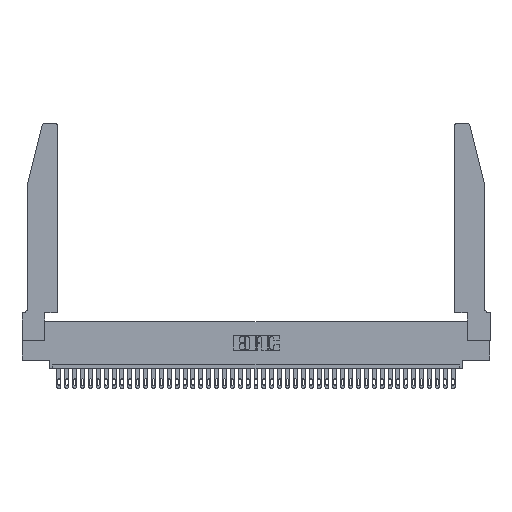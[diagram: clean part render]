
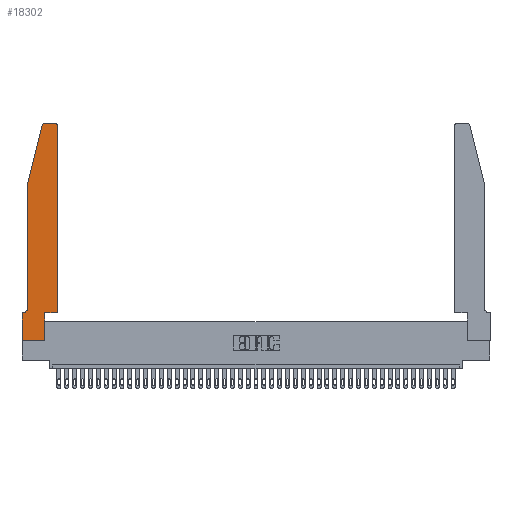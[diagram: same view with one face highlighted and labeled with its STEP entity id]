
A CAD part, top view. The second image highlights one B-rep face of the part: STEP entity #18302.
In plain terms, the highlighted planar face has unit normal (0, 0, 1).
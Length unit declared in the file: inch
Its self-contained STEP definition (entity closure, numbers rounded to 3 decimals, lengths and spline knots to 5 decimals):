
#527 = CARTESIAN_POINT ( 'NONE',  ( 0.0755, 2., 0.37 ) ) ;
#579 = DIRECTION ( 'NONE',  ( 1., 0., 0. ) ) ;
#668 = DIRECTION ( 'NONE',  ( -0.239, -0.971, 0. ) ) ;
#1017 = LINE ( 'NONE', #32076, #15274 ) ;
#1327 = VERTEX_POINT ( 'NONE', #15235 ) ;
#2550 = CIRCLE ( 'NONE', #15860, 0.07 ) ;
#3714 = VECTOR ( 'NONE', #8068, 39.37008 ) ;
#3719 = EDGE_CURVE ( 'NONE', #20723, #32697, #11274, .T. ) ;
#4238 = VERTEX_POINT ( 'NONE', #23955 ) ;
#4839 = EDGE_CURVE ( 'NONE', #19956, #35145, #35488, .T. ) ;
#6407 = VERTEX_POINT ( 'NONE', #12222 ) ;
#6591 = DIRECTION ( 'NONE',  ( 1., 0., 0. ) ) ;
#6674 = ORIENTED_EDGE ( 'NONE', *, *, #29566, .T. ) ;
#7957 = FACE_OUTER_BOUND ( 'NONE', #36875, .T. ) ;
#8068 = DIRECTION ( 'NONE',  ( 0., -1., 0. ) ) ;
#8104 = ORIENTED_EDGE ( 'NONE', *, *, #24002, .T. ) ;
#8950 = EDGE_CURVE ( 'NONE', #16561, #6407, #25975, .T. ) ;
#9251 = CARTESIAN_POINT ( 'NONE',  ( 0., 0.35, 0.37 ) ) ;
#9753 = ORIENTED_EDGE ( 'NONE', *, *, #22561, .T. ) ;
#11274 = LINE ( 'NONE', #40471, #36041 ) ;
#12089 = DIRECTION ( 'NONE',  ( 1., 0., 0. ) ) ;
#12222 = CARTESIAN_POINT ( 'NONE',  ( 0.0755, 2., 0.37 ) ) ;
#14002 = CARTESIAN_POINT ( 'NONE',  ( 0., 0.35, 0.37 ) ) ;
#14170 = LINE ( 'NONE', #36055, #40534 ) ;
#14314 = CIRCLE ( 'NONE', #27351, 0.03 ) ;
#14444 = ORIENTED_EDGE ( 'NONE', *, *, #4839, .T. ) ;
#14509 = DIRECTION ( 'NONE',  ( 0., 1., 0. ) ) ;
#14653 = CARTESIAN_POINT ( 'NONE',  ( 0.284, 2.75, 0.37 ) ) ;
#14959 = ORIENTED_EDGE ( 'NONE', *, *, #37560, .T. ) ;
#15235 = CARTESIAN_POINT ( 'NONE',  ( 0.0055, 0.35, 0.37 ) ) ;
#15274 = VECTOR ( 'NONE', #31943, 39.37008 ) ;
#15860 = AXIS2_PLACEMENT_3D ( 'NONE', #17059, #26700, #26286 ) ;
#16427 = PLANE ( 'NONE',  #25209 ) ;
#16561 = VERTEX_POINT ( 'NONE', #34721 ) ;
#16781 = AXIS2_PLACEMENT_3D ( 'NONE', #28694, #24999, #24856 ) ;
#17059 = CARTESIAN_POINT ( 'NONE',  ( 0.0055, 0.42, 0.37 ) ) ;
#18076 = CARTESIAN_POINT ( 'NONE',  ( 0.0755, 0.42, 0.37 ) ) ;
#18302 = ADVANCED_FACE ( 'NONE', ( #7957 ), #16427, .T. ) ;
#18661 = DIRECTION ( 'NONE',  ( -1., 0., 0. ) ) ;
#19955 = VERTEX_POINT ( 'NONE', #18076 ) ;
#19956 = VERTEX_POINT ( 'NONE', #31541 ) ;
#19989 = CARTESIAN_POINT ( 'NONE',  ( 0.4205, 2.72, 0.37 ) ) ;
#20416 = ORIENTED_EDGE ( 'NONE', *, *, #34501, .T. ) ;
#20723 = VERTEX_POINT ( 'NONE', #20806 ) ;
#20806 = CARTESIAN_POINT ( 'NONE',  ( 0.4205, 2.75, 0.37 ) ) ;
#20946 = VERTEX_POINT ( 'NONE', #39478 ) ;
#22561 = EDGE_CURVE ( 'NONE', #23092, #20946, #34065, .T. ) ;
#23092 = VERTEX_POINT ( 'NONE', #33394 ) ;
#23416 = DIRECTION ( 'NONE',  ( 0., 0., 1. ) ) ;
#23955 = CARTESIAN_POINT ( 'NONE',  ( 0.2865, 0.35, 0.37 ) ) ;
#24002 = EDGE_CURVE ( 'NONE', #32697, #16561, #32438, .T. ) ;
#24856 = DIRECTION ( 'NONE',  ( 1., 0., 0. ) ) ;
#24986 = LINE ( 'NONE', #30204, #3714 ) ;
#24999 = DIRECTION ( 'NONE',  ( 0., 0., 1. ) ) ;
#25209 = AXIS2_PLACEMENT_3D ( 'NONE', #14002, #40057, #12089 ) ;
#25975 = LINE ( 'NONE', #527, #39612 ) ;
#26286 = DIRECTION ( 'NONE',  ( -1., 0., 0. ) ) ;
#26387 = DIRECTION ( 'NONE',  ( -1., 0., 0. ) ) ;
#26432 = LINE ( 'NONE', #26812, #26969 ) ;
#26700 = DIRECTION ( 'NONE',  ( 0., 0., -1. ) ) ;
#26812 = CARTESIAN_POINT ( 'NONE',  ( 0.2865, 0.35, 0.37 ) ) ;
#26825 = VECTOR ( 'NONE', #27560, 39.37008 ) ;
#26969 = VECTOR ( 'NONE', #14509, 39.37008 ) ;
#27351 = AXIS2_PLACEMENT_3D ( 'NONE', #19989, #23416, #579 ) ;
#27560 = DIRECTION ( 'NONE',  ( 0., 1., 0. ) ) ;
#28401 = ORIENTED_EDGE ( 'NONE', *, *, #3719, .T. ) ;
#28591 = CARTESIAN_POINT ( 'NONE',  ( 0.0755, 0.35, 0.37 ) ) ;
#28694 = CARTESIAN_POINT ( 'NONE',  ( 0.284, 2.72, 0.37 ) ) ;
#28917 = EDGE_CURVE ( 'NONE', #4238, #19956, #1017, .T. ) ;
#29566 = EDGE_CURVE ( 'NONE', #30030, #23092, #14170, .T. ) ;
#29856 = ORIENTED_EDGE ( 'NONE', *, *, #28917, .T. ) ;
#30030 = VERTEX_POINT ( 'NONE', #9251 ) ;
#30204 = CARTESIAN_POINT ( 'NONE',  ( 0.0755, 2., 0.37 ) ) ;
#30359 = CARTESIAN_POINT ( 'NONE',  ( 0.4505, 0.35, 0.37 ) ) ;
#31541 = CARTESIAN_POINT ( 'NONE',  ( 0.4505, 0.35, 0.37 ) ) ;
#31943 = DIRECTION ( 'NONE',  ( 1., 0., 0. ) ) ;
#32076 = CARTESIAN_POINT ( 'NONE',  ( 0.4505, 0.35, 0.37 ) ) ;
#32438 = CIRCLE ( 'NONE', #16781, 0.03 ) ;
#32697 = VERTEX_POINT ( 'NONE', #14653 ) ;
#32760 = ORIENTED_EDGE ( 'NONE', *, *, #8950, .T. ) ;
#33196 = ORIENTED_EDGE ( 'NONE', *, *, #34432, .T. ) ;
#33394 = CARTESIAN_POINT ( 'NONE',  ( 0., 0., 0.37 ) ) ;
#34065 = LINE ( 'NONE', #40951, #37081 ) ;
#34337 = EDGE_CURVE ( 'NONE', #35145, #20723, #14314, .T. ) ;
#34432 = EDGE_CURVE ( 'NONE', #6407, #19955, #24986, .T. ) ;
#34501 = EDGE_CURVE ( 'NONE', #20946, #4238, #26432, .T. ) ;
#34644 = VECTOR ( 'NONE', #26387, 39.37008 ) ;
#34721 = CARTESIAN_POINT ( 'NONE',  ( 0.25487, 2.72718, 0.37 ) ) ;
#35145 = VERTEX_POINT ( 'NONE', #38482 ) ;
#35488 = LINE ( 'NONE', #30359, #26825 ) ;
#36041 = VECTOR ( 'NONE', #18661, 39.37008 ) ;
#36055 = CARTESIAN_POINT ( 'NONE',  ( 0., 0., 0.37 ) ) ;
#36875 = EDGE_LOOP ( 'NONE', ( #28401, #8104, #32760, #33196, #40166, #14959, #6674, #9753, #20416, #29856, #14444, #38155 ) ) ;
#37081 = VECTOR ( 'NONE', #6591, 39.37008 ) ;
#37560 = EDGE_CURVE ( 'NONE', #1327, #30030, #39108, .T. ) ;
#38155 = ORIENTED_EDGE ( 'NONE', *, *, #34337, .T. ) ;
#38482 = CARTESIAN_POINT ( 'NONE',  ( 0.4505, 2.72, 0.37 ) ) ;
#39108 = LINE ( 'NONE', #28591, #34644 ) ;
#39165 = DIRECTION ( 'NONE',  ( 0., -1., 0. ) ) ;
#39478 = CARTESIAN_POINT ( 'NONE',  ( 0.2865, 0., 0.37 ) ) ;
#39612 = VECTOR ( 'NONE', #668, 39.37008 ) ;
#39624 = EDGE_CURVE ( 'NONE', #19955, #1327, #2550, .T. ) ;
#40057 = DIRECTION ( 'NONE',  ( 0., 0., 1. ) ) ;
#40166 = ORIENTED_EDGE ( 'NONE', *, *, #39624, .T. ) ;
#40471 = CARTESIAN_POINT ( 'NONE',  ( 0.2605, 2.75, 0.37 ) ) ;
#40534 = VECTOR ( 'NONE', #39165, 39.37008 ) ;
#40951 = CARTESIAN_POINT ( 'NONE',  ( 0., 0., 0.37 ) ) ;
